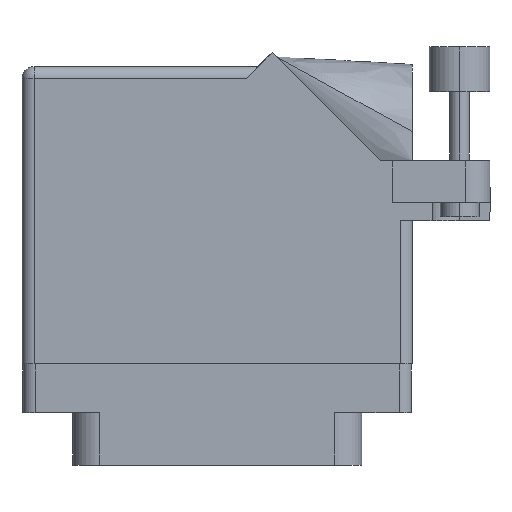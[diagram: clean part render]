
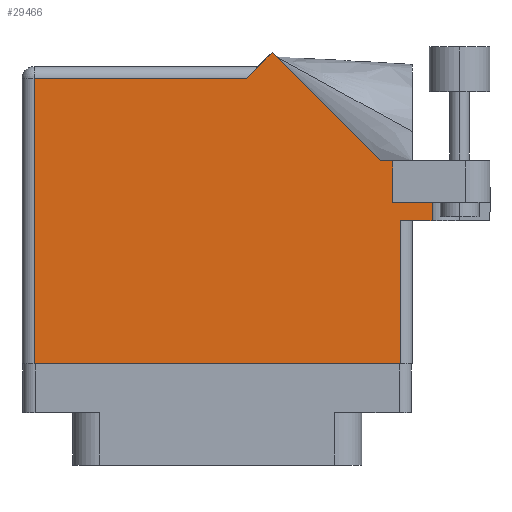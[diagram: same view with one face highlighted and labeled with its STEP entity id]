
A CAD part, front view. The second image highlights one B-rep face of the part: STEP entity #29466.
In plain terms, the highlighted face is planar.
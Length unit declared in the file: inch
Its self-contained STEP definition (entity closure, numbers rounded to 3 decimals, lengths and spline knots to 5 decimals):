
#15 = LINE ( 'NONE', #30311, #1976 ) ;
#378 = CARTESIAN_POINT ( 'NONE',  ( 0.905, 0.731, 0.455 ) ) ;
#391 = VERTEX_POINT ( 'NONE', #8570 ) ;
#814 = EDGE_CURVE ( 'NONE', #13455, #9628, #1771, .T. ) ;
#1037 = CARTESIAN_POINT ( 'NONE',  ( 0.943, 0.637, 0.455 ) ) ;
#1417 = ORIENTED_EDGE ( 'NONE', *, *, #12130, .T. ) ;
#1771 = LINE ( 'NONE', #14375, #10570 ) ;
#1976 = VECTOR ( 'NONE', #39863, 39.37008 ) ;
#2198 = ORIENTED_EDGE ( 'NONE', *, *, #26049, .F. ) ;
#2887 = EDGE_CURVE ( 'NONE', #9628, #16387, #39515, .T. ) ;
#3667 = EDGE_CURVE ( 'NONE', #18119, #36020, #35056, .T. ) ;
#4064 = VECTOR ( 'NONE', #9607, 39.37008 ) ;
#4832 = VECTOR ( 'NONE', #34278, 39.37008 ) ;
#5280 = DIRECTION ( 'NONE',  ( 0., -1., 0. ) ) ;
#6126 = PLANE ( 'NONE',  #38539 ) ;
#6385 = VECTOR ( 'NONE', #7711, 39.37008 ) ;
#6490 = CARTESIAN_POINT ( 'NONE',  ( 0.28271, 1.50071, 0.455 ) ) ;
#6531 = CARTESIAN_POINT ( 'NONE',  ( -1.005, 1.43, 0.455 ) ) ;
#6863 = VECTOR ( 'NONE', #18677, 39.37008 ) ;
#7185 = EDGE_CURVE ( 'NONE', #36020, #27042, #40087, .T. ) ;
#7711 = DIRECTION ( 'NONE',  ( -0.707, 0.707, 0. ) ) ;
#7830 = LINE ( 'NONE', #35485, #6385 ) ;
#8290 = DIRECTION ( 'NONE',  ( -1., 0., 0. ) ) ;
#8570 = CARTESIAN_POINT ( 'NONE',  ( 1.1065, 0.731, 0.455 ) ) ;
#9381 = CARTESIAN_POINT ( 'NONE',  ( 1.005, 0.637, 0.455 ) ) ;
#9535 = CARTESIAN_POINT ( 'NONE',  ( 0.905, 0.731, 0.455 ) ) ;
#9607 = DIRECTION ( 'NONE',  ( -1., 0., 0. ) ) ;
#9628 = VERTEX_POINT ( 'NONE', #37404 ) ;
#9694 = DIRECTION ( 'NONE',  ( 0., 0., -1. ) ) ;
#10570 = VECTOR ( 'NONE', #39472, 39.37008 ) ;
#11090 = VERTEX_POINT ( 'NONE', #378 ) ;
#11216 = EDGE_CURVE ( 'NONE', #16994, #18119, #7830, .T. ) ;
#11695 = VECTOR ( 'NONE', #5280, 39.37008 ) ;
#12130 = EDGE_CURVE ( 'NONE', #27042, #13455, #15, .T. ) ;
#12273 = EDGE_CURVE ( 'NONE', #11090, #23648, #16101, .T. ) ;
#12865 = ORIENTED_EDGE ( 'NONE', *, *, #27556, .T. ) ;
#12879 = EDGE_CURVE ( 'NONE', #391, #20036, #25363, .T. ) ;
#13003 = CARTESIAN_POINT ( 'NONE',  ( 0.905, 0.731, 0.455 ) ) ;
#13455 = VERTEX_POINT ( 'NONE', #26483 ) ;
#13632 = VECTOR ( 'NONE', #20889, 39.37008 ) ;
#13824 = DIRECTION ( 'NONE',  ( -0.707, -0.707, 0. ) ) ;
#14375 = CARTESIAN_POINT ( 'NONE',  ( -1.005, -0.1, 0.455 ) ) ;
#14497 = CARTESIAN_POINT ( 'NONE',  ( -0.943, 1.368, 0.455 ) ) ;
#14726 = EDGE_LOOP ( 'NONE', ( #38720, #22465, #22258, #38390, #2198, #21698, #12865, #38957, #16960, #39810, #1417 ) ) ;
#16011 = VECTOR ( 'NONE', #13824, 39.37008 ) ;
#16101 = LINE ( 'NONE', #9535, #4832 ) ;
#16387 = VERTEX_POINT ( 'NONE', #1037 ) ;
#16960 = ORIENTED_EDGE ( 'NONE', *, *, #3667, .T. ) ;
#16994 = VERTEX_POINT ( 'NONE', #35513 ) ;
#17841 = CARTESIAN_POINT ( 'NONE',  ( 1.1065, 1.06177, 0.455 ) ) ;
#17847 = VECTOR ( 'NONE', #25434, 39.37008 ) ;
#18009 = EDGE_CURVE ( 'NONE', #16387, #20036, #26452, .T. ) ;
#18119 = VERTEX_POINT ( 'NONE', #6490 ) ;
#18677 = DIRECTION ( 'NONE',  ( 1., 0., 0. ) ) ;
#20036 = VERTEX_POINT ( 'NONE', #33622 ) ;
#20889 = DIRECTION ( 'NONE',  ( 0., 1., 0. ) ) ;
#21698 = ORIENTED_EDGE ( 'NONE', *, *, #12273, .T. ) ;
#22258 = ORIENTED_EDGE ( 'NONE', *, *, #18009, .T. ) ;
#22465 = ORIENTED_EDGE ( 'NONE', *, *, #2887, .T. ) ;
#22621 = LINE ( 'NONE', #31029, #4064 ) ;
#23489 = FACE_OUTER_BOUND ( 'NONE', #14726, .T. ) ;
#23648 = VERTEX_POINT ( 'NONE', #37101 ) ;
#25363 = LINE ( 'NONE', #17841, #11695 ) ;
#25434 = DIRECTION ( 'NONE',  ( 1., 0., 0. ) ) ;
#26049 = EDGE_CURVE ( 'NONE', #11090, #391, #26175, .T. ) ;
#26175 = LINE ( 'NONE', #13003, #17847 ) ;
#26452 = LINE ( 'NONE', #9381, #6863 ) ;
#26483 = CARTESIAN_POINT ( 'NONE',  ( -0.943, -0.1, 0.455 ) ) ;
#27042 = VERTEX_POINT ( 'NONE', #14497 ) ;
#27556 = EDGE_CURVE ( 'NONE', #23648, #16994, #22621, .T. ) ;
#29378 = CARTESIAN_POINT ( 'NONE',  ( 0.212, 1.43, 0.455 ) ) ;
#29466 = ADVANCED_FACE ( 'NONE', ( #23489 ), #6126, .F. ) ;
#29825 = CARTESIAN_POINT ( 'NONE',  ( -1.005, 1.368, 0.455 ) ) ;
#30196 = CARTESIAN_POINT ( 'NONE',  ( 0.15, 1.368, 0.455 ) ) ;
#30311 = CARTESIAN_POINT ( 'NONE',  ( -0.943, -0.1, 0.455 ) ) ;
#31029 = CARTESIAN_POINT ( 'NONE',  ( 1.405, 0.944, 0.455 ) ) ;
#33622 = CARTESIAN_POINT ( 'NONE',  ( 1.1065, 0.637, 0.455 ) ) ;
#34278 = DIRECTION ( 'NONE',  ( 0., 1., 0. ) ) ;
#34707 = DIRECTION ( 'NONE',  ( -1., 0., 0. ) ) ;
#35056 = LINE ( 'NONE', #29378, #16011 ) ;
#35485 = CARTESIAN_POINT ( 'NONE',  ( 0.83942, 0.944, 0.455 ) ) ;
#35513 = CARTESIAN_POINT ( 'NONE',  ( 0.83942, 0.944, 0.455 ) ) ;
#36020 = VERTEX_POINT ( 'NONE', #30196 ) ;
#37101 = CARTESIAN_POINT ( 'NONE',  ( 0.905, 0.944, 0.455 ) ) ;
#37404 = CARTESIAN_POINT ( 'NONE',  ( 0.943, -0.1, 0.455 ) ) ;
#38390 = ORIENTED_EDGE ( 'NONE', *, *, #12879, .F. ) ;
#38539 = AXIS2_PLACEMENT_3D ( 'NONE', #6531, #9694, #34707 ) ;
#38720 = ORIENTED_EDGE ( 'NONE', *, *, #814, .T. ) ;
#38957 = ORIENTED_EDGE ( 'NONE', *, *, #11216, .T. ) ;
#39104 = VECTOR ( 'NONE', #8290, 39.37008 ) ;
#39472 = DIRECTION ( 'NONE',  ( 1., 0., 0. ) ) ;
#39515 = LINE ( 'NONE', #39600, #13632 ) ;
#39600 = CARTESIAN_POINT ( 'NONE',  ( 0.943, 0.637, 0.455 ) ) ;
#39810 = ORIENTED_EDGE ( 'NONE', *, *, #7185, .T. ) ;
#39863 = DIRECTION ( 'NONE',  ( 0., -1., 0. ) ) ;
#40087 = LINE ( 'NONE', #29825, #39104 ) ;
